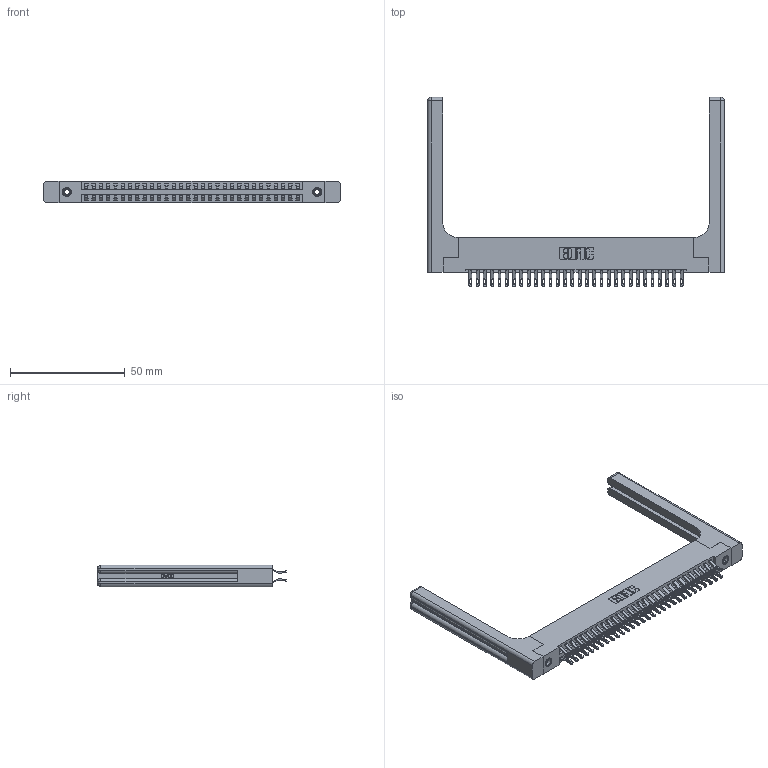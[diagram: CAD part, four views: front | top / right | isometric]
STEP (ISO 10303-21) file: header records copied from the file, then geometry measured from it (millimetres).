
FILE_DESCRIPTION (( 'STEP AP203' ), '1' );
FILE_NAME ('346-060-555-258.STEP', '2022-05-21T11:50:38', ( '' ), ( '' ), 'SwSTEP 2.0', 'SolidWorks 2020', '' );
FILE_SCHEMA (( 'CONFIG_CONTROL_DESIGN' ));
Length unit declared in the file: inch
Products named in the file (5): 346 Part_Flush Mounting Lugs - 0.156 Dia-TH; 345-250-001_345-250-001-102; 346-220-058_345-220-058; 346-060-555-258; 345-292-001_555 Tail
Assembly tree (65 placements, depth 2):
  346-060-555-258
    346 Part_Flush Mounting Lugs - 0.156 Dia-TH
    345-292-001_555 Tail  x60
    345-250-001_345-250-001-102  x2
    346-220-058_345-220-058  x2
Bounding box: 129.31 x 82.42 x 9.4 mm (x, y, z)
Volume: 20166.4 mm3; surface area: 22857.9 mm2
Topology: 65 solids, 65 shells, 3872 faces, 12011 edges, 7986 vertices
Faces by surface type: plane 2218, cylinder 1594, bspline 36, cone 12, sphere 8, torus 4
Entity records: 27118 total; most frequent: CARTESIAN_POINT 5533, ORIENTED_EDGE 4232, DIRECTION 3828, EDGE_CURVE 2116, VECTOR 1752, LINE 1752, VERTEX_POINT 1402, AXIS2_PLACEMENT_3D 1038
